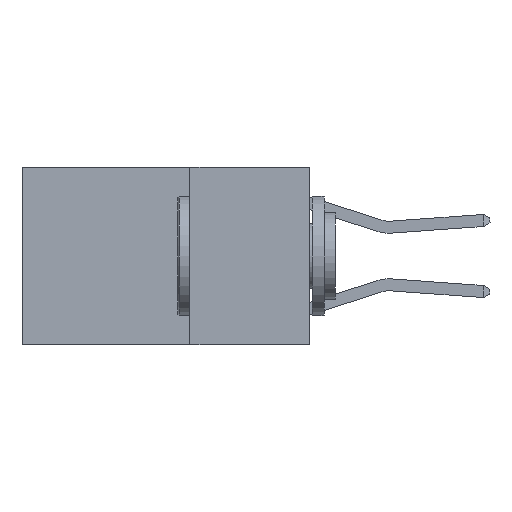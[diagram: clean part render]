
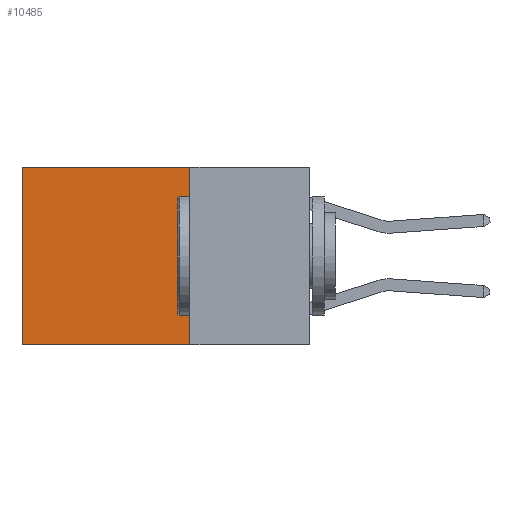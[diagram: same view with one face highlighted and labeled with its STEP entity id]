
A CAD part, left-side view. The second image highlights one B-rep face of the part: STEP entity #10485.
In plain terms, the highlighted planar face has unit normal (-1, 0, 0).
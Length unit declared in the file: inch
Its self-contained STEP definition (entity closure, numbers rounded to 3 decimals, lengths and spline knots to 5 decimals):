
#265 = VERTEX_POINT ( 'NONE', #18552 ) ;
#1093 = VERTEX_POINT ( 'NONE', #6825 ) ;
#2536 = EDGE_CURVE ( 'NONE', #19486, #1093, #5955, .T. ) ;
#2576 = AXIS2_PLACEMENT_3D ( 'NONE', #14332, #3646, #16086 ) ;
#3001 = DIRECTION ( 'NONE',  ( 0., 1., 0. ) ) ;
#3646 = DIRECTION ( 'NONE',  ( 1., 0., 0. ) ) ;
#5955 = LINE ( 'NONE', #9493, #19607 ) ;
#6584 = VECTOR ( 'NONE', #3001, 39.37008 ) ;
#6825 = CARTESIAN_POINT ( 'NONE',  ( 0.2625, 0.6, 0. ) ) ;
#6862 = EDGE_CURVE ( 'NONE', #19705, #265, #11352, .T. ) ;
#7170 = PLANE ( 'NONE',  #2576 ) ;
#7639 = VECTOR ( 'NONE', #8571, 39.37008 ) ;
#8571 = DIRECTION ( 'NONE',  ( 0., 0., -1. ) ) ;
#8629 = ORIENTED_EDGE ( 'NONE', *, *, #6862, .F. ) ;
#8904 = DIRECTION ( 'NONE',  ( 0., 0., -1. ) ) ;
#9493 = CARTESIAN_POINT ( 'NONE',  ( 0.2625, 0.25, 0. ) ) ;
#10485 = ADVANCED_FACE ( 'NONE', ( #15168 ), #7170, .F. ) ;
#11352 = LINE ( 'NONE', #17177, #6584 ) ;
#11962 = LINE ( 'NONE', #12488, #16680 ) ;
#12275 = EDGE_CURVE ( 'NONE', #1093, #265, #17094, .T. ) ;
#12354 = CARTESIAN_POINT ( 'NONE',  ( 0.2625, 0.25, -0.37 ) ) ;
#12488 = CARTESIAN_POINT ( 'NONE',  ( 0.2625, 0.25, 0. ) ) ;
#12539 = EDGE_LOOP ( 'NONE', ( #18591, #8629, #14280, #12813 ) ) ;
#12813 = ORIENTED_EDGE ( 'NONE', *, *, #2536, .T. ) ;
#13598 = CARTESIAN_POINT ( 'NONE',  ( 0.2625, 0.25, 0. ) ) ;
#13849 = CARTESIAN_POINT ( 'NONE',  ( 0.2625, 0.6, 0. ) ) ;
#14280 = ORIENTED_EDGE ( 'NONE', *, *, #14873, .F. ) ;
#14332 = CARTESIAN_POINT ( 'NONE',  ( 0.2625, 0.25, 0. ) ) ;
#14873 = EDGE_CURVE ( 'NONE', #19486, #19705, #11962, .T. ) ;
#15168 = FACE_OUTER_BOUND ( 'NONE', #12539, .T. ) ;
#16086 = DIRECTION ( 'NONE',  ( 0., 0., -1. ) ) ;
#16680 = VECTOR ( 'NONE', #8904, 39.37008 ) ;
#17094 = LINE ( 'NONE', #13849, #7639 ) ;
#17177 = CARTESIAN_POINT ( 'NONE',  ( 0.2625, 0.25, -0.37 ) ) ;
#18552 = CARTESIAN_POINT ( 'NONE',  ( 0.2625, 0.6, -0.37 ) ) ;
#18591 = ORIENTED_EDGE ( 'NONE', *, *, #12275, .T. ) ;
#19486 = VERTEX_POINT ( 'NONE', #13598 ) ;
#19607 = VECTOR ( 'NONE', #20163, 39.37008 ) ;
#19705 = VERTEX_POINT ( 'NONE', #12354 ) ;
#20163 = DIRECTION ( 'NONE',  ( 0., 1., 0. ) ) ;
